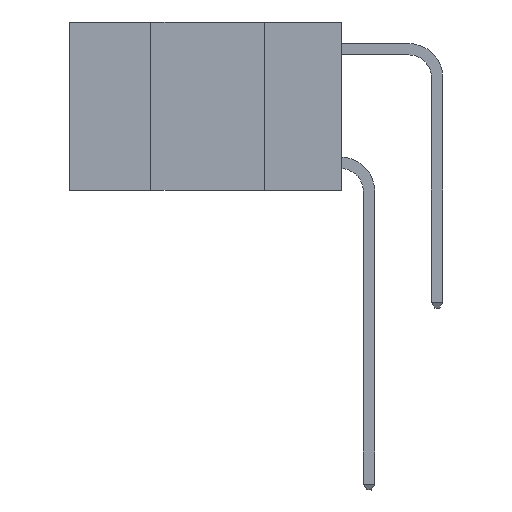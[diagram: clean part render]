
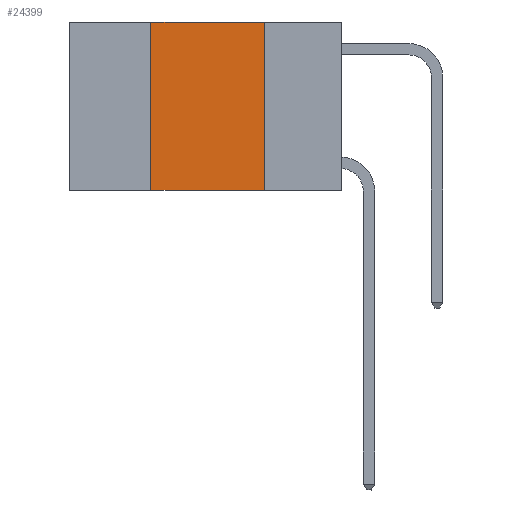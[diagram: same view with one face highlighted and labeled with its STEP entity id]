
A CAD part, left-side view. The second image highlights one B-rep face of the part: STEP entity #24399.
In plain terms, the highlighted planar face has unit normal (-1, 0, 0).
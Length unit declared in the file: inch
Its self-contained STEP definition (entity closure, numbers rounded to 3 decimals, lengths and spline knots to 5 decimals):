
#655 = CARTESIAN_POINT ( 'NONE',  ( 0., 0.42, 0. ) ) ;
#982 = CARTESIAN_POINT ( 'NONE',  ( 0., 0.17, -0.37 ) ) ;
#1153 = DIRECTION ( 'NONE',  ( 0., 0., -1. ) ) ;
#1388 = LINE ( 'NONE', #3504, #7554 ) ;
#1672 = VERTEX_POINT ( 'NONE', #15640 ) ;
#2031 = CARTESIAN_POINT ( 'NONE',  ( 0., 0.6, 0. ) ) ;
#3504 = CARTESIAN_POINT ( 'NONE',  ( 0., 0.6, -0.37 ) ) ;
#3772 = VERTEX_POINT ( 'NONE', #10103 ) ;
#3843 = ORIENTED_EDGE ( 'NONE', *, *, #13551, .F. ) ;
#3997 = VECTOR ( 'NONE', #14477, 39.37008 ) ;
#4592 = DIRECTION ( 'NONE',  ( 0., 0., -1. ) ) ;
#5208 = EDGE_CURVE ( 'NONE', #3772, #26745, #1388, .T. ) ;
#5828 = CARTESIAN_POINT ( 'NONE',  ( 0., 0.17, 0. ) ) ;
#6393 = LINE ( 'NONE', #16011, #10048 ) ;
#7554 = VECTOR ( 'NONE', #12668, 39.37008 ) ;
#8050 = VECTOR ( 'NONE', #1153, 39.37008 ) ;
#8156 = ORIENTED_EDGE ( 'NONE', *, *, #10518, .F. ) ;
#10048 = VECTOR ( 'NONE', #27214, 39.37008 ) ;
#10103 = CARTESIAN_POINT ( 'NONE',  ( 0., 0.42, -0.37 ) ) ;
#10518 = EDGE_CURVE ( 'NONE', #1672, #26745, #19381, .T. ) ;
#12668 = DIRECTION ( 'NONE',  ( 0., -1., 0. ) ) ;
#13551 = EDGE_CURVE ( 'NONE', #3772, #24154, #16036, .T. ) ;
#14477 = DIRECTION ( 'NONE',  ( 0., 0., 1. ) ) ;
#15640 = CARTESIAN_POINT ( 'NONE',  ( 0., 0.17, 0. ) ) ;
#16011 = CARTESIAN_POINT ( 'NONE',  ( 0., 0.6, 0. ) ) ;
#16036 = LINE ( 'NONE', #655, #3997 ) ;
#18117 = PLANE ( 'NONE',  #27413 ) ;
#19381 = LINE ( 'NONE', #5828, #8050 ) ;
#20401 = DIRECTION ( 'NONE',  ( 1., 0., 0. ) ) ;
#22037 = ORIENTED_EDGE ( 'NONE', *, *, #24332, .F. ) ;
#23247 = EDGE_LOOP ( 'NONE', ( #8156, #22037, #3843, #23516 ) ) ;
#23516 = ORIENTED_EDGE ( 'NONE', *, *, #5208, .T. ) ;
#24154 = VERTEX_POINT ( 'NONE', #25721 ) ;
#24332 = EDGE_CURVE ( 'NONE', #24154, #1672, #6393, .T. ) ;
#24399 = ADVANCED_FACE ( 'NONE', ( #25384 ), #18117, .F. ) ;
#25384 = FACE_OUTER_BOUND ( 'NONE', #23247, .T. ) ;
#25721 = CARTESIAN_POINT ( 'NONE',  ( 0., 0.42, 0. ) ) ;
#26745 = VERTEX_POINT ( 'NONE', #982 ) ;
#27214 = DIRECTION ( 'NONE',  ( 0., -1., 0. ) ) ;
#27413 = AXIS2_PLACEMENT_3D ( 'NONE', #2031, #20401, #4592 ) ;
